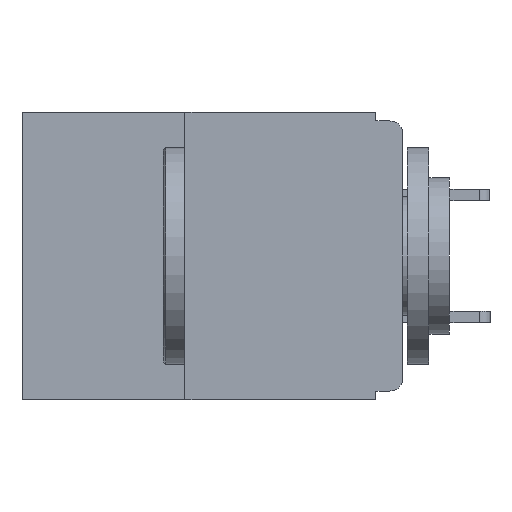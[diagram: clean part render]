
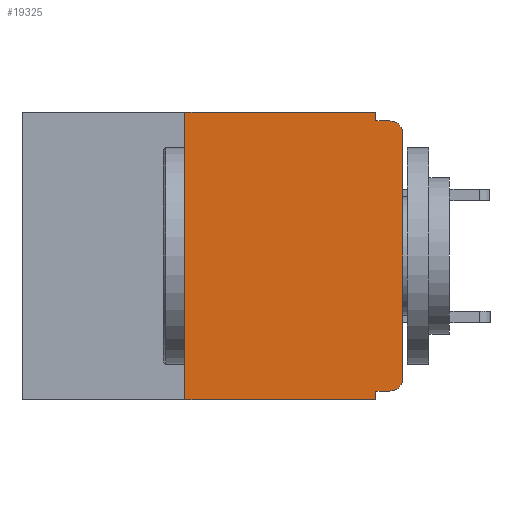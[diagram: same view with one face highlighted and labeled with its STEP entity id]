
A CAD part, left-side view. The second image highlights one B-rep face of the part: STEP entity #19325.
In plain terms, the highlighted planar face has unit normal (-1, 0, 0).
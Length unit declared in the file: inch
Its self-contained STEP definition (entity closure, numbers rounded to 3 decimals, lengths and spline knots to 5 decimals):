
#218 = EDGE_CURVE ( 'NONE', #27367, #2757, #29594, .T. ) ;
#230 = VERTEX_POINT ( 'NONE', #13719 ) ;
#414 = VERTEX_POINT ( 'NONE', #21326 ) ;
#541 = CARTESIAN_POINT ( 'NONE',  ( 0., 0.031, -0.33 ) ) ;
#874 = VERTEX_POINT ( 'NONE', #28272 ) ;
#2674 = DIRECTION ( 'NONE',  ( 0., 0., -1. ) ) ;
#2757 = VERTEX_POINT ( 'NONE', #27902 ) ;
#2786 = LINE ( 'NONE', #12111, #29728 ) ;
#3046 = EDGE_CURVE ( 'NONE', #19310, #9451, #9377, .T. ) ;
#3434 = CIRCLE ( 'NONE', #26683, 0.015 ) ;
#4155 = CARTESIAN_POINT ( 'NONE',  ( 0., 0.437, 0. ) ) ;
#4197 = PLANE ( 'NONE',  #22422 ) ;
#4397 = EDGE_CURVE ( 'NONE', #27367, #230, #2786, .T. ) ;
#4509 = LINE ( 'NONE', #17635, #31380 ) ;
#4569 = DIRECTION ( 'NONE',  ( 0., 0., 1. ) ) ;
#4732 = CARTESIAN_POINT ( 'NONE',  ( 0., 0.015, -0.01 ) ) ;
#4992 = DIRECTION ( 'NONE',  ( 0., 0., 1. ) ) ;
#6849 = DIRECTION ( 'NONE',  ( 1., 0., 0. ) ) ;
#7282 = ORIENTED_EDGE ( 'NONE', *, *, #30962, .F. ) ;
#7930 = CARTESIAN_POINT ( 'NONE',  ( 0., 0.031, -0.33 ) ) ;
#9377 = LINE ( 'NONE', #14263, #28580 ) ;
#9451 = VERTEX_POINT ( 'NONE', #541 ) ;
#9685 = EDGE_CURVE ( 'NONE', #414, #23020, #19429, .T. ) ;
#10911 = ORIENTED_EDGE ( 'NONE', *, *, #21607, .F. ) ;
#11680 = DIRECTION ( 'NONE',  ( 0., 0., -1. ) ) ;
#12111 = CARTESIAN_POINT ( 'NONE',  ( 0., 0., -0.32 ) ) ;
#12409 = DIRECTION ( 'NONE',  ( -1., 0., 0. ) ) ;
#12453 = VECTOR ( 'NONE', #4992, 39.37008 ) ;
#12461 = VECTOR ( 'NONE', #25043, 39.37008 ) ;
#12626 = EDGE_CURVE ( 'NONE', #874, #20069, #20900, .T. ) ;
#12983 = ORIENTED_EDGE ( 'NONE', *, *, #30867, .T. ) ;
#13395 = CARTESIAN_POINT ( 'NONE',  ( 0., 0., -0.01 ) ) ;
#13719 = CARTESIAN_POINT ( 'NONE',  ( 0., 0.031, -0.32 ) ) ;
#14263 = CARTESIAN_POINT ( 'NONE',  ( 0., 0.437, -0.33 ) ) ;
#14516 = CARTESIAN_POINT ( 'NONE',  ( 0., 0.437, 0. ) ) ;
#16037 = DIRECTION ( 'NONE',  ( 0., -1., 0. ) ) ;
#16075 = DIRECTION ( 'NONE',  ( -1., 0., 0. ) ) ;
#16115 = CARTESIAN_POINT ( 'NONE',  ( 0., 0.015, -0.305 ) ) ;
#16134 = VECTOR ( 'NONE', #2674, 39.37008 ) ;
#16459 = DIRECTION ( 'NONE',  ( 0., 0., -1. ) ) ;
#17571 = ORIENTED_EDGE ( 'NONE', *, *, #4397, .F. ) ;
#17635 = CARTESIAN_POINT ( 'NONE',  ( 0., 0., 0. ) ) ;
#18891 = EDGE_CURVE ( 'NONE', #2757, #30349, #4509, .T. ) ;
#19310 = VERTEX_POINT ( 'NONE', #19775 ) ;
#19325 = ADVANCED_FACE ( 'NONE', ( #24482 ), #4197, .F. ) ;
#19429 = LINE ( 'NONE', #4155, #12461 ) ;
#19775 = CARTESIAN_POINT ( 'NONE',  ( 0., 0.25, -0.33 ) ) ;
#19941 = ORIENTED_EDGE ( 'NONE', *, *, #12626, .F. ) ;
#19982 = DIRECTION ( 'NONE',  ( 0., 1., 0. ) ) ;
#20069 = VERTEX_POINT ( 'NONE', #4732 ) ;
#20519 = LINE ( 'NONE', #27298, #33342 ) ;
#20900 = LINE ( 'NONE', #13395, #26179 ) ;
#20905 = CARTESIAN_POINT ( 'NONE',  ( 0., 0., -0.025 ) ) ;
#21326 = CARTESIAN_POINT ( 'NONE',  ( 0., 0.25, 0. ) ) ;
#21607 = EDGE_CURVE ( 'NONE', #23020, #874, #20519, .T. ) ;
#22422 = AXIS2_PLACEMENT_3D ( 'NONE', #14516, #6849, #25090 ) ;
#22823 = ORIENTED_EDGE ( 'NONE', *, *, #31074, .F. ) ;
#23020 = VERTEX_POINT ( 'NONE', #23107 ) ;
#23107 = CARTESIAN_POINT ( 'NONE',  ( 0., 0.031, 0. ) ) ;
#24331 = EDGE_LOOP ( 'NONE', ( #32053, #12983, #19941, #10911, #33199, #7282, #30487, #22823, #17571, #26101 ) ) ;
#24482 = FACE_OUTER_BOUND ( 'NONE', #24331, .T. ) ;
#25029 = CARTESIAN_POINT ( 'NONE',  ( 0., 0.015, -0.32 ) ) ;
#25043 = DIRECTION ( 'NONE',  ( 0., -1., 0. ) ) ;
#25090 = DIRECTION ( 'NONE',  ( 0., 0., -1. ) ) ;
#25864 = CARTESIAN_POINT ( 'NONE',  ( 0., 0.25, -0.33 ) ) ;
#26101 = ORIENTED_EDGE ( 'NONE', *, *, #218, .T. ) ;
#26179 = VECTOR ( 'NONE', #16037, 39.37008 ) ;
#26683 = AXIS2_PLACEMENT_3D ( 'NONE', #28043, #12409, #30599 ) ;
#27132 = LINE ( 'NONE', #25864, #12453 ) ;
#27298 = CARTESIAN_POINT ( 'NONE',  ( 0., 0.031, 0. ) ) ;
#27367 = VERTEX_POINT ( 'NONE', #25029 ) ;
#27902 = CARTESIAN_POINT ( 'NONE',  ( 0., 0., -0.305 ) ) ;
#28032 = AXIS2_PLACEMENT_3D ( 'NONE', #16115, #16075, #16459 ) ;
#28043 = CARTESIAN_POINT ( 'NONE',  ( 0., 0.015, -0.025 ) ) ;
#28272 = CARTESIAN_POINT ( 'NONE',  ( 0., 0.031, -0.01 ) ) ;
#28580 = VECTOR ( 'NONE', #31287, 39.37008 ) ;
#29594 = CIRCLE ( 'NONE', #28032, 0.015 ) ;
#29728 = VECTOR ( 'NONE', #19982, 39.37008 ) ;
#29951 = LINE ( 'NONE', #7930, #16134 ) ;
#30349 = VERTEX_POINT ( 'NONE', #20905 ) ;
#30487 = ORIENTED_EDGE ( 'NONE', *, *, #3046, .T. ) ;
#30599 = DIRECTION ( 'NONE',  ( 0., 0., -1. ) ) ;
#30867 = EDGE_CURVE ( 'NONE', #30349, #20069, #3434, .T. ) ;
#30962 = EDGE_CURVE ( 'NONE', #19310, #414, #27132, .T. ) ;
#31074 = EDGE_CURVE ( 'NONE', #230, #9451, #29951, .T. ) ;
#31287 = DIRECTION ( 'NONE',  ( 0., -1., 0. ) ) ;
#31380 = VECTOR ( 'NONE', #4569, 39.37008 ) ;
#32053 = ORIENTED_EDGE ( 'NONE', *, *, #18891, .T. ) ;
#33199 = ORIENTED_EDGE ( 'NONE', *, *, #9685, .F. ) ;
#33342 = VECTOR ( 'NONE', #11680, 39.37008 ) ;
